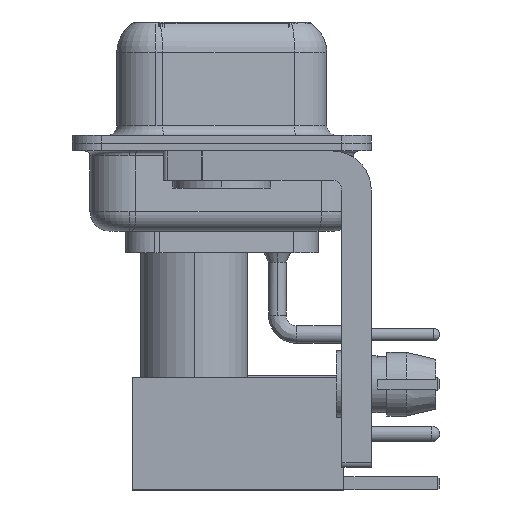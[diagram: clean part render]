
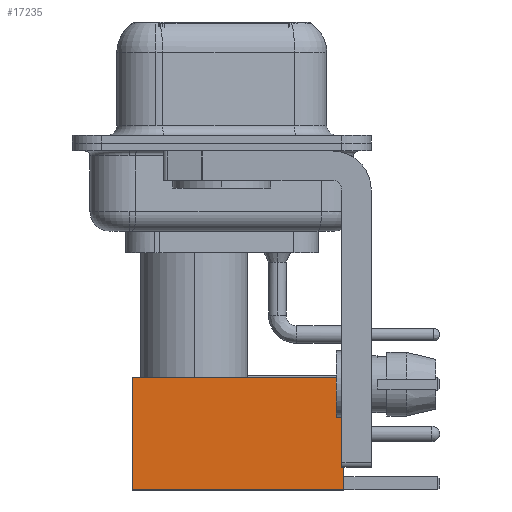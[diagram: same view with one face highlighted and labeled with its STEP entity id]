
A CAD part, left-side view. The second image highlights one B-rep face of the part: STEP entity #17235.
In plain terms, the highlighted face is planar.
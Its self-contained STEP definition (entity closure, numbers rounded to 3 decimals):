
#277 = DIRECTION ( 'NONE',  ( 0., 0., 1. ) ) ;
#2041 = VECTOR ( 'NONE', #30963, 1000. ) ;
#2474 = CARTESIAN_POINT ( 'NONE',  ( 2.875, 2.875, 0. ) ) ;
#4629 = VECTOR ( 'NONE', #5890, 1000. ) ;
#5112 = ORIENTED_EDGE ( 'NONE', *, *, #26926, .T. ) ;
#5480 = FACE_OUTER_BOUND ( 'NONE', #37169, .T. ) ;
#5647 = CARTESIAN_POINT ( 'NONE',  ( 2.875, 2.875, 10.82 ) ) ;
#5835 = EDGE_CURVE ( 'NONE', #38954, #6092, #12467, .T. ) ;
#5890 = DIRECTION ( 'NONE',  ( -1., 0., 0. ) ) ;
#5906 = ORIENTED_EDGE ( 'NONE', *, *, #5835, .F. ) ;
#5975 = EDGE_CURVE ( 'NONE', #6092, #38034, #37836, .T. ) ;
#6092 = VERTEX_POINT ( 'NONE', #30278 ) ;
#7475 = DIRECTION ( 'NONE',  ( 0., 0., -1. ) ) ;
#12453 = PLANE ( 'NONE',  #13089 ) ;
#12467 = LINE ( 'NONE', #15857, #4629 ) ;
#13089 = AXIS2_PLACEMENT_3D ( 'NONE', #2474, #21258, #277 ) ;
#14148 = CARTESIAN_POINT ( 'NONE',  ( -2.875, 2.875, 0. ) ) ;
#14859 = VECTOR ( 'NONE', #7475, 1000. ) ;
#15179 = CARTESIAN_POINT ( 'NONE',  ( 2.875, 2.875, 0. ) ) ;
#15857 = CARTESIAN_POINT ( 'NONE',  ( 0., 2.875, 10.82 ) ) ;
#17235 = ADVANCED_FACE ( 'NONE', ( #5480 ), #12453, .T. ) ;
#19089 = ORIENTED_EDGE ( 'NONE', *, *, #23146, .T. ) ;
#20305 = VECTOR ( 'NONE', #38198, 1000. ) ;
#20896 = VERTEX_POINT ( 'NONE', #23873 ) ;
#21258 = DIRECTION ( 'NONE',  ( 0., 1., 0. ) ) ;
#22646 = CARTESIAN_POINT ( 'NONE',  ( -2.875, 2.875, 0. ) ) ;
#23146 = EDGE_CURVE ( 'NONE', #20896, #38034, #38588, .T. ) ;
#23873 = CARTESIAN_POINT ( 'NONE',  ( 2.875, 2.875, 0. ) ) ;
#24425 = ORIENTED_EDGE ( 'NONE', *, *, #5975, .F. ) ;
#26000 = CARTESIAN_POINT ( 'NONE',  ( 0., 2.875, 0. ) ) ;
#26926 = EDGE_CURVE ( 'NONE', #38954, #20896, #36564, .T. ) ;
#30278 = CARTESIAN_POINT ( 'NONE',  ( -2.875, 2.875, 10.82 ) ) ;
#30963 = DIRECTION ( 'NONE',  ( 0., 0., -1. ) ) ;
#36564 = LINE ( 'NONE', #15179, #2041 ) ;
#37169 = EDGE_LOOP ( 'NONE', ( #5112, #19089, #24425, #5906 ) ) ;
#37836 = LINE ( 'NONE', #22646, #14859 ) ;
#38034 = VERTEX_POINT ( 'NONE', #14148 ) ;
#38198 = DIRECTION ( 'NONE',  ( -1., 0., 0. ) ) ;
#38588 = LINE ( 'NONE', #26000, #20305 ) ;
#38954 = VERTEX_POINT ( 'NONE', #5647 ) ;
